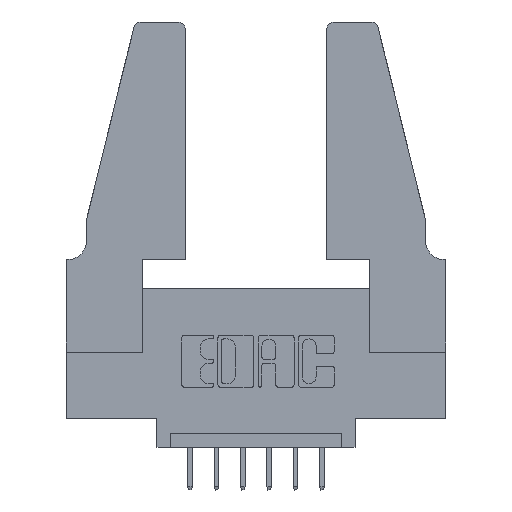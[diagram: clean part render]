
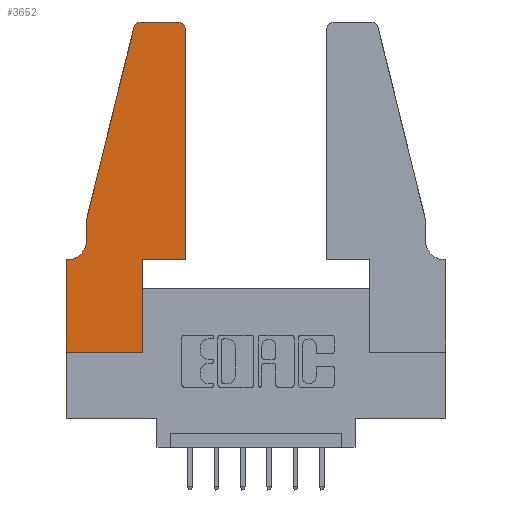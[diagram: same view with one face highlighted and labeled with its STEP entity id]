
A CAD part, top view. The second image highlights one B-rep face of the part: STEP entity #3652.
In plain terms, the highlighted planar face has unit normal (0, 0, 1).
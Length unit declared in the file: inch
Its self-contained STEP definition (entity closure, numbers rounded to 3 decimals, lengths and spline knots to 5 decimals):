
#21 = LINE ( 'NONE', #9023, #4262 ) ;
#216 = VERTEX_POINT ( 'NONE', #8650 ) ;
#291 = DIRECTION ( 'NONE',  ( 1., 0., 0. ) ) ;
#331 = CIRCLE ( 'NONE', #1349, 0.03 ) ;
#420 = VECTOR ( 'NONE', #11383, 39.37008 ) ;
#454 = CARTESIAN_POINT ( 'NONE',  ( 0.4505, 1.22, 0.37 ) ) ;
#544 = VERTEX_POINT ( 'NONE', #6665 ) ;
#863 = AXIS2_PLACEMENT_3D ( 'NONE', #4215, #4145, #9655 ) ;
#875 = CIRCLE ( 'NONE', #9916, 0.03 ) ;
#944 = ORIENTED_EDGE ( 'NONE', *, *, #4046, .T. ) ;
#1246 = DIRECTION ( 'NONE',  ( 0., 0., 1. ) ) ;
#1301 = VERTEX_POINT ( 'NONE', #6851 ) ;
#1349 = AXIS2_PLACEMENT_3D ( 'NONE', #9858, #10815, #10773 ) ;
#2141 = CARTESIAN_POINT ( 'NONE',  ( 0.25487, 1.22718, 0.37 ) ) ;
#2514 = EDGE_LOOP ( 'NONE', ( #5302, #6720, #4647, #10946, #4037, #8113, #9158, #944, #4426, #4680, #7204, #3011 ) ) ;
#2652 = CARTESIAN_POINT ( 'NONE',  ( 0.4505, 0.35, 0.37 ) ) ;
#2709 = CARTESIAN_POINT ( 'NONE',  ( 0., 0., 0.37 ) ) ;
#2839 = DIRECTION ( 'NONE',  ( 1., 0., 0. ) ) ;
#3011 = ORIENTED_EDGE ( 'NONE', *, *, #4534, .T. ) ;
#3027 = EDGE_CURVE ( 'NONE', #3897, #10308, #5939, .T. ) ;
#3121 = PLANE ( 'NONE',  #9527 ) ;
#3412 = EDGE_CURVE ( 'NONE', #10308, #8390, #4041, .T. ) ;
#3457 = LINE ( 'NONE', #2709, #4598 ) ;
#3478 = EDGE_CURVE ( 'NONE', #216, #1301, #8459, .T. ) ;
#3612 = VECTOR ( 'NONE', #8255, 39.37008 ) ;
#3632 = EDGE_CURVE ( 'NONE', #10530, #544, #10861, .T. ) ;
#3652 = ADVANCED_FACE ( 'NONE', ( #5474 ), #3121, .T. ) ;
#3671 = CARTESIAN_POINT ( 'NONE',  ( 0.0755, 0.5, 0.37 ) ) ;
#3897 = VERTEX_POINT ( 'NONE', #3671 ) ;
#4037 = ORIENTED_EDGE ( 'NONE', *, *, #3412, .T. ) ;
#4041 = CIRCLE ( 'NONE', #863, 0.07 ) ;
#4046 = EDGE_CURVE ( 'NONE', #5266, #216, #3457, .T. ) ;
#4145 = DIRECTION ( 'NONE',  ( 0., 0., -1. ) ) ;
#4215 = CARTESIAN_POINT ( 'NONE',  ( 0.0055, 0.42, 0.37 ) ) ;
#4262 = VECTOR ( 'NONE', #10015, 39.37008 ) ;
#4426 = ORIENTED_EDGE ( 'NONE', *, *, #3478, .T. ) ;
#4534 = EDGE_CURVE ( 'NONE', #10654, #10530, #331, .T. ) ;
#4589 = DIRECTION ( 'NONE',  ( 0., 0., 1. ) ) ;
#4598 = VECTOR ( 'NONE', #291, 39.37008 ) ;
#4647 = ORIENTED_EDGE ( 'NONE', *, *, #5596, .T. ) ;
#4680 = ORIENTED_EDGE ( 'NONE', *, *, #9379, .T. ) ;
#4846 = LINE ( 'NONE', #5358, #11499 ) ;
#5266 = VERTEX_POINT ( 'NONE', #8392 ) ;
#5302 = ORIENTED_EDGE ( 'NONE', *, *, #3632, .T. ) ;
#5358 = CARTESIAN_POINT ( 'NONE',  ( 0.0755, 0.35, 0.37 ) ) ;
#5474 = FACE_OUTER_BOUND ( 'NONE', #2514, .T. ) ;
#5494 = DIRECTION ( 'NONE',  ( 0., -1., 0. ) ) ;
#5509 = DIRECTION ( 'NONE',  ( 1., 0., 0. ) ) ;
#5531 = CARTESIAN_POINT ( 'NONE',  ( 0.0055, 0.35, 0.37 ) ) ;
#5593 = EDGE_CURVE ( 'NONE', #544, #10572, #875, .T. ) ;
#5596 = EDGE_CURVE ( 'NONE', #10572, #3897, #21, .T. ) ;
#5707 = CARTESIAN_POINT ( 'NONE',  ( 0., 0., 0.37 ) ) ;
#5939 = LINE ( 'NONE', #7415, #9737 ) ;
#5942 = DIRECTION ( 'NONE',  ( 1., 0., 0. ) ) ;
#5969 = VECTOR ( 'NONE', #10840, 39.37008 ) ;
#6220 = CARTESIAN_POINT ( 'NONE',  ( 0.0755, 0.42, 0.37 ) ) ;
#6575 = VECTOR ( 'NONE', #5942, 39.37008 ) ;
#6657 = EDGE_CURVE ( 'NONE', #9835, #5266, #11193, .T. ) ;
#6659 = CARTESIAN_POINT ( 'NONE',  ( 0., 0.35, 0.37 ) ) ;
#6665 = CARTESIAN_POINT ( 'NONE',  ( 0.284, 1.25, 0.37 ) ) ;
#6720 = ORIENTED_EDGE ( 'NONE', *, *, #5593, .T. ) ;
#6851 = CARTESIAN_POINT ( 'NONE',  ( 0.2865, 0.35, 0.37 ) ) ;
#7204 = ORIENTED_EDGE ( 'NONE', *, *, #11579, .T. ) ;
#7415 = CARTESIAN_POINT ( 'NONE',  ( 0.0755, 0.5, 0.37 ) ) ;
#8113 = ORIENTED_EDGE ( 'NONE', *, *, #9055, .T. ) ;
#8255 = DIRECTION ( 'NONE',  ( -1., 0., 0. ) ) ;
#8390 = VERTEX_POINT ( 'NONE', #5531 ) ;
#8392 = CARTESIAN_POINT ( 'NONE',  ( 0., 0., 0.37 ) ) ;
#8459 = LINE ( 'NONE', #9914, #9006 ) ;
#8650 = CARTESIAN_POINT ( 'NONE',  ( 0.2865, 0., 0.37 ) ) ;
#9006 = VECTOR ( 'NONE', #11584, 39.37008 ) ;
#9023 = CARTESIAN_POINT ( 'NONE',  ( 0.0755, 0.5, 0.37 ) ) ;
#9055 = EDGE_CURVE ( 'NONE', #8390, #9835, #4846, .T. ) ;
#9061 = CARTESIAN_POINT ( 'NONE',  ( 0.284, 1.22, 0.37 ) ) ;
#9158 = ORIENTED_EDGE ( 'NONE', *, *, #6657, .T. ) ;
#9379 = EDGE_CURVE ( 'NONE', #1301, #10908, #11355, .T. ) ;
#9527 = AXIS2_PLACEMENT_3D ( 'NONE', #11172, #1246, #2839 ) ;
#9555 = CARTESIAN_POINT ( 'NONE',  ( 0.4505, 0.35, 0.37 ) ) ;
#9655 = DIRECTION ( 'NONE',  ( -1., 0., 0. ) ) ;
#9737 = VECTOR ( 'NONE', #5494, 39.37008 ) ;
#9835 = VERTEX_POINT ( 'NONE', #6659 ) ;
#9858 = CARTESIAN_POINT ( 'NONE',  ( 0.4205, 1.22, 0.37 ) ) ;
#9914 = CARTESIAN_POINT ( 'NONE',  ( 0.2865, 0.35, 0.37 ) ) ;
#9916 = AXIS2_PLACEMENT_3D ( 'NONE', #9061, #4589, #5509 ) ;
#9992 = CARTESIAN_POINT ( 'NONE',  ( 0.2605, 1.25, 0.37 ) ) ;
#10015 = DIRECTION ( 'NONE',  ( -0.239, -0.971, 0. ) ) ;
#10229 = DIRECTION ( 'NONE',  ( -1., 0., 0. ) ) ;
#10308 = VERTEX_POINT ( 'NONE', #6220 ) ;
#10530 = VERTEX_POINT ( 'NONE', #11090 ) ;
#10572 = VERTEX_POINT ( 'NONE', #2141 ) ;
#10587 = CARTESIAN_POINT ( 'NONE',  ( 0.4505, 0.35, 0.37 ) ) ;
#10625 = LINE ( 'NONE', #2652, #5969 ) ;
#10654 = VERTEX_POINT ( 'NONE', #454 ) ;
#10773 = DIRECTION ( 'NONE',  ( 1., 0., 0. ) ) ;
#10815 = DIRECTION ( 'NONE',  ( 0., 0., 1. ) ) ;
#10840 = DIRECTION ( 'NONE',  ( 0., 1., 0. ) ) ;
#10861 = LINE ( 'NONE', #9992, #3612 ) ;
#10908 = VERTEX_POINT ( 'NONE', #10587 ) ;
#10946 = ORIENTED_EDGE ( 'NONE', *, *, #3027, .T. ) ;
#11090 = CARTESIAN_POINT ( 'NONE',  ( 0.4205, 1.25, 0.37 ) ) ;
#11172 = CARTESIAN_POINT ( 'NONE',  ( 0., 0.35, 0.37 ) ) ;
#11193 = LINE ( 'NONE', #5707, #420 ) ;
#11355 = LINE ( 'NONE', #9555, #6575 ) ;
#11383 = DIRECTION ( 'NONE',  ( 0., -1., 0. ) ) ;
#11499 = VECTOR ( 'NONE', #10229, 39.37008 ) ;
#11579 = EDGE_CURVE ( 'NONE', #10908, #10654, #10625, .T. ) ;
#11584 = DIRECTION ( 'NONE',  ( 0., 1., 0. ) ) ;
